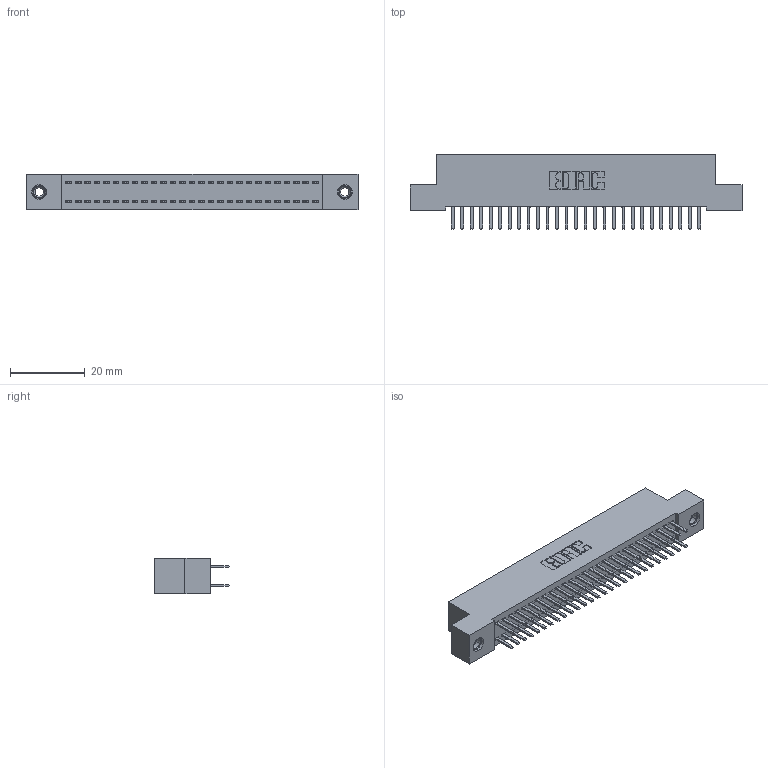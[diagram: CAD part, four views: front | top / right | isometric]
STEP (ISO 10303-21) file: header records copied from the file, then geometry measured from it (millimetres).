
FILE_DESCRIPTION (( 'STEP AP203' ), '1' );
FILE_NAME ('392-054-520-208.STEP', '2018-08-17T08:09:31', ( '' ), ( '' ), 'SwSTEP 2.0', 'SolidWorks 2016', '' );
FILE_SCHEMA (( 'CONFIG_CONTROL_DESIGN' ));
Length unit declared in the file: inch
Products named in the file (4): 342 Part_TI; 345-292-001_345-293-120; 345-250-001_345-250-003-102; 392-054-520-208
Assembly tree (57 placements, depth 2):
  392-054-520-208
    342 Part_TI
    345-292-001_345-293-120  x54
    345-250-001_345-250-003-102  x2
Bounding box: 88.9 x 20.02 x 9.4 mm (x, y, z)
Volume: 7887.2 mm3; surface area: 12423.1 mm2
Topology: 57 solids, 57 shells, 3194 faces, 9237 edges, 6006 vertices
Faces by surface type: plane 2150, cylinder 1028, cone 12, torus 4
Entity records: 20478 total; most frequent: CARTESIAN_POINT 3405, ORIENTED_EDGE 3322, DIRECTION 2955, EDGE_CURVE 1661, VECTOR 1509, LINE 1509, VERTEX_POINT 1100, AXIS2_PLACEMENT_3D 723
